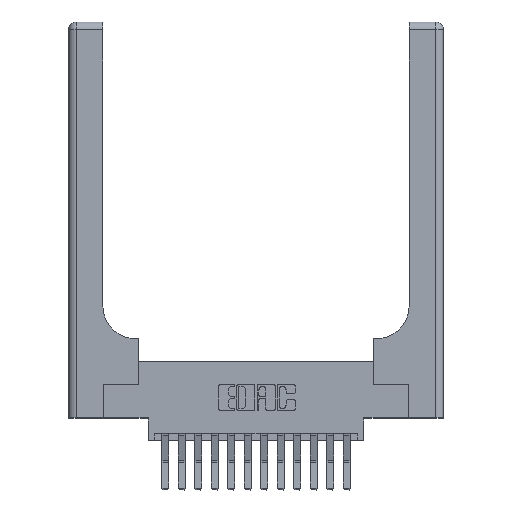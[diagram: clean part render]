
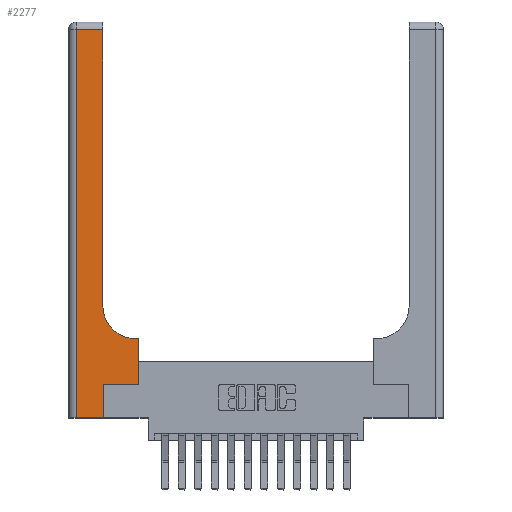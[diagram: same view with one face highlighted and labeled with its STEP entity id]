
A CAD part, top view. The second image highlights one B-rep face of the part: STEP entity #2277.
In plain terms, the highlighted planar face has unit normal (0, 0, 1).
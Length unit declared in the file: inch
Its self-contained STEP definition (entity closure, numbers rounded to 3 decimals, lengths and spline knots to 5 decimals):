
#431 = VERTEX_POINT ( 'NONE', #10390 ) ;
#762 = CARTESIAN_POINT ( 'NONE',  ( 0.26, 0.85, 0.37 ) ) ;
#861 = VECTOR ( 'NONE', #3270, 39.37008 ) ;
#1155 = CARTESIAN_POINT ( 'NONE',  ( 0.528, 0.25, 0.37 ) ) ;
#1870 = DIRECTION ( 'NONE',  ( -1., 0., 0. ) ) ;
#2277 = ADVANCED_FACE ( 'NONE', ( #15034 ), #13393, .F. ) ;
#2489 = VERTEX_POINT ( 'NONE', #12589 ) ;
#2889 = LINE ( 'NONE', #14233, #16298 ) ;
#3093 = ORIENTED_EDGE ( 'NONE', *, *, #17168, .T. ) ;
#3270 = DIRECTION ( 'NONE',  ( -1., 0., 0. ) ) ;
#3400 = CARTESIAN_POINT ( 'NONE',  ( 0., 0., 0.37 ) ) ;
#3811 = ORIENTED_EDGE ( 'NONE', *, *, #4317, .T. ) ;
#4317 = EDGE_CURVE ( 'NONE', #9279, #431, #4422, .T. ) ;
#4422 = LINE ( 'NONE', #8555, #15581 ) ;
#4827 = LINE ( 'NONE', #11702, #15139 ) ;
#4956 = DIRECTION ( 'NONE',  ( 1., 0., 0. ) ) ;
#5413 = LINE ( 'NONE', #10837, #8054 ) ;
#6553 = CARTESIAN_POINT ( 'NONE',  ( 0.265, 0., 0.37 ) ) ;
#7047 = LINE ( 'NONE', #15254, #7435 ) ;
#7149 = ORIENTED_EDGE ( 'NONE', *, *, #11354, .T. ) ;
#7201 = DIRECTION ( 'NONE',  ( 0., 0., -1. ) ) ;
#7435 = VECTOR ( 'NONE', #13794, 39.37008 ) ;
#7783 = CARTESIAN_POINT ( 'NONE',  ( 0.265, 0.25, 0.37 ) ) ;
#7893 = EDGE_CURVE ( 'NONE', #12619, #10155, #8171, .T. ) ;
#8054 = VECTOR ( 'NONE', #13543, 39.37008 ) ;
#8113 = CARTESIAN_POINT ( 'NONE',  ( 0.528, 0.6, 0.37 ) ) ;
#8171 = LINE ( 'NONE', #6553, #11102 ) ;
#8249 = CARTESIAN_POINT ( 'NONE',  ( 0., 3., 0.37 ) ) ;
#8355 = EDGE_CURVE ( 'NONE', #12787, #13745, #13041, .T. ) ;
#8456 = CARTESIAN_POINT ( 'NONE',  ( 0.51, 0.85, 0.37 ) ) ;
#8528 = ORIENTED_EDGE ( 'NONE', *, *, #15027, .T. ) ;
#8555 = CARTESIAN_POINT ( 'NONE',  ( 0., 2.94, 0.37 ) ) ;
#9074 = CARTESIAN_POINT ( 'NONE',  ( 0.26, 2.94, 0.37 ) ) ;
#9279 = VERTEX_POINT ( 'NONE', #9074 ) ;
#9284 = DIRECTION ( 'NONE',  ( 0., 0., -1. ) ) ;
#9463 = ORIENTED_EDGE ( 'NONE', *, *, #15080, .T. ) ;
#9781 = AXIS2_PLACEMENT_3D ( 'NONE', #8249, #9284, #17697 ) ;
#10002 = DIRECTION ( 'NONE',  ( 1., 0., 0. ) ) ;
#10147 = LINE ( 'NONE', #15548, #861 ) ;
#10155 = VERTEX_POINT ( 'NONE', #7783 ) ;
#10283 = LINE ( 'NONE', #3400, #10610 ) ;
#10300 = CARTESIAN_POINT ( 'NONE',  ( 0.265, 0., 0.37 ) ) ;
#10390 = CARTESIAN_POINT ( 'NONE',  ( 0.06, 2.94, 0.37 ) ) ;
#10610 = VECTOR ( 'NONE', #4956, 39.37008 ) ;
#10837 = CARTESIAN_POINT ( 'NONE',  ( 0.26, 3., 0.37 ) ) ;
#10878 = DIRECTION ( 'NONE',  ( 0., 1., 0. ) ) ;
#11102 = VECTOR ( 'NONE', #10878, 39.37008 ) ;
#11354 = EDGE_CURVE ( 'NONE', #431, #2489, #4827, .T. ) ;
#11659 = DIRECTION ( 'NONE',  ( 1., 0., 0. ) ) ;
#11702 = CARTESIAN_POINT ( 'NONE',  ( 0.06, 3., 0.37 ) ) ;
#12589 = CARTESIAN_POINT ( 'NONE',  ( 0.06, 0., 0.37 ) ) ;
#12619 = VERTEX_POINT ( 'NONE', #10300 ) ;
#12787 = VERTEX_POINT ( 'NONE', #16144 ) ;
#13010 = ORIENTED_EDGE ( 'NONE', *, *, #8355, .T. ) ;
#13037 = EDGE_CURVE ( 'NONE', #2489, #12619, #10283, .T. ) ;
#13041 = CIRCLE ( 'NONE', #17043, 0.25 ) ;
#13393 = PLANE ( 'NONE',  #9781 ) ;
#13543 = DIRECTION ( 'NONE',  ( 0., 1., 0. ) ) ;
#13745 = VERTEX_POINT ( 'NONE', #762 ) ;
#13794 = DIRECTION ( 'NONE',  ( 0., 1., 0. ) ) ;
#13893 = VERTEX_POINT ( 'NONE', #8113 ) ;
#14233 = CARTESIAN_POINT ( 'NONE',  ( 0.265, 0.25, 0.37 ) ) ;
#14781 = EDGE_LOOP ( 'NONE', ( #9463, #3811, #7149, #15362, #15986, #3093, #17447, #8528, #13010 ) ) ;
#15027 = EDGE_CURVE ( 'NONE', #13893, #12787, #10147, .T. ) ;
#15034 = FACE_OUTER_BOUND ( 'NONE', #14781, .T. ) ;
#15080 = EDGE_CURVE ( 'NONE', #13745, #9279, #5413, .T. ) ;
#15139 = VECTOR ( 'NONE', #17138, 39.37008 ) ;
#15254 = CARTESIAN_POINT ( 'NONE',  ( 0.528, 0.25, 0.37 ) ) ;
#15362 = ORIENTED_EDGE ( 'NONE', *, *, #13037, .T. ) ;
#15548 = CARTESIAN_POINT ( 'NONE',  ( 0.26, 0.6, 0.37 ) ) ;
#15581 = VECTOR ( 'NONE', #1870, 39.37008 ) ;
#15986 = ORIENTED_EDGE ( 'NONE', *, *, #7893, .T. ) ;
#16144 = CARTESIAN_POINT ( 'NONE',  ( 0.51, 0.6, 0.37 ) ) ;
#16298 = VECTOR ( 'NONE', #11659, 39.37008 ) ;
#17043 = AXIS2_PLACEMENT_3D ( 'NONE', #8456, #7201, #10002 ) ;
#17079 = EDGE_CURVE ( 'NONE', #17387, #13893, #7047, .T. ) ;
#17138 = DIRECTION ( 'NONE',  ( 0., -1., 0. ) ) ;
#17168 = EDGE_CURVE ( 'NONE', #10155, #17387, #2889, .T. ) ;
#17387 = VERTEX_POINT ( 'NONE', #1155 ) ;
#17447 = ORIENTED_EDGE ( 'NONE', *, *, #17079, .T. ) ;
#17697 = DIRECTION ( 'NONE',  ( -1., 0., 0. ) ) ;
